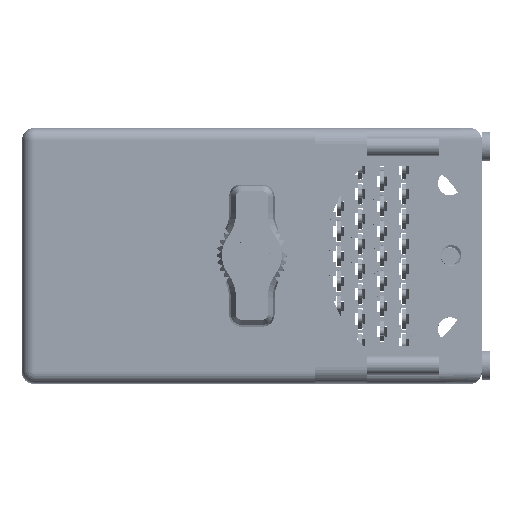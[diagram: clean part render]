
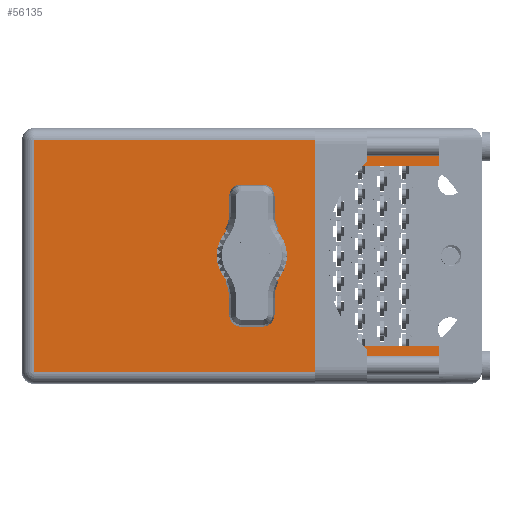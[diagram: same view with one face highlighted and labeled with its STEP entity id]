
A CAD part, top view. The second image highlights one B-rep face of the part: STEP entity #56135.
In plain terms, the highlighted face is planar.
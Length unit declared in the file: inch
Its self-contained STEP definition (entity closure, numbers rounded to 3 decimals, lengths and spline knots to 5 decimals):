
#214 = LINE ( 'NONE', #39672, #83314 ) ;
#845 = VERTEX_POINT ( 'NONE', #43709 ) ;
#1133 = EDGE_CURVE ( 'NONE', #43625, #47633, #113852, .T. ) ;
#6510 = DIRECTION ( 'NONE',  ( 0., 1., 0. ) ) ;
#6665 = EDGE_LOOP ( 'NONE', ( #37885, #8141 ) ) ;
#8141 = ORIENTED_EDGE ( 'NONE', *, *, #75667, .F. ) ;
#11729 = ORIENTED_EDGE ( 'NONE', *, *, #46398, .T. ) ;
#15214 = CIRCLE ( 'NONE', #17256, 0.17 ) ;
#16119 = CARTESIAN_POINT ( 'NONE',  ( 0., 2.03, -1.46 ) ) ;
#16270 = VECTOR ( 'NONE', #66486, 39.37008 ) ;
#17256 = AXIS2_PLACEMENT_3D ( 'NONE', #53500, #71880, #35400 ) ;
#17842 = CARTESIAN_POINT ( 'NONE',  ( 0.07, 2.03, -0.07 ) ) ;
#19711 = VERTEX_POINT ( 'NONE', #57983 ) ;
#20556 = EDGE_CURVE ( 'NONE', #73441, #50418, #86297, .T. ) ;
#21620 = CIRCLE ( 'NONE', #43722, 0.17 ) ;
#24631 = VECTOR ( 'NONE', #107066, 39.37008 ) ;
#25936 = ORIENTED_EDGE ( 'NONE', *, *, #43017, .T. ) ;
#27123 = VECTOR ( 'NONE', #75668, 39.37008 ) ;
#32045 = CARTESIAN_POINT ( 'NONE',  ( 2.499, 2.03, -1.46 ) ) ;
#35400 = DIRECTION ( 'NONE',  ( 0., 0., 1. ) ) ;
#35811 = ORIENTED_EDGE ( 'NONE', *, *, #83329, .T. ) ;
#37885 = ORIENTED_EDGE ( 'NONE', *, *, #70931, .F. ) ;
#38828 = CARTESIAN_POINT ( 'NONE',  ( 2.499, 2.03, -0.07 ) ) ;
#39672 = CARTESIAN_POINT ( 'NONE',  ( 1.785, 2.03, -1.305 ) ) ;
#40812 = FACE_BOUND ( 'NONE', #6665, .T. ) ;
#43017 = EDGE_CURVE ( 'NONE', #55716, #47633, #66844, .T. ) ;
#43625 = VERTEX_POINT ( 'NONE', #32045 ) ;
#43709 = CARTESIAN_POINT ( 'NONE',  ( 1.3775, 2.03, -0.935 ) ) ;
#43722 = AXIS2_PLACEMENT_3D ( 'NONE', #115340, #49992, #114144 ) ;
#46033 = VECTOR ( 'NONE', #117172, 39.37008 ) ;
#46398 = EDGE_CURVE ( 'NONE', #49380, #82780, #96384, .T. ) ;
#47633 = VERTEX_POINT ( 'NONE', #61844 ) ;
#49380 = VERTEX_POINT ( 'NONE', #49765 ) ;
#49470 = FACE_OUTER_BOUND ( 'NONE', #64217, .T. ) ;
#49765 = CARTESIAN_POINT ( 'NONE',  ( 0.07, 2.03, -1.46 ) ) ;
#49992 = DIRECTION ( 'NONE',  ( 0., 1., 0. ) ) ;
#50418 = VERTEX_POINT ( 'NONE', #77451 ) ;
#53500 = CARTESIAN_POINT ( 'NONE',  ( 1.3775, 2.03, -0.765 ) ) ;
#55258 = CARTESIAN_POINT ( 'NONE',  ( 2.499, 2.03, -0.225 ) ) ;
#55716 = VERTEX_POINT ( 'NONE', #75066 ) ;
#56135 = ADVANCED_FACE ( 'NONE', ( #49470, #40812 ), #116376, .T. ) ;
#57983 = CARTESIAN_POINT ( 'NONE',  ( 1.785, 2.03, -0.225 ) ) ;
#61399 = CARTESIAN_POINT ( 'NONE',  ( 0., 2.03, -1.53 ) ) ;
#61844 = CARTESIAN_POINT ( 'NONE',  ( 2.499, 2.03, -1.305 ) ) ;
#64217 = EDGE_LOOP ( 'NONE', ( #11729, #109467, #86239, #91679, #83997, #25936, #95914, #35811 ) ) ;
#66486 = DIRECTION ( 'NONE',  ( 0., 0., 1. ) ) ;
#66844 = LINE ( 'NONE', #75076, #104107 ) ;
#70622 = DIRECTION ( 'NONE',  ( 0., 0., 1. ) ) ;
#70931 = EDGE_CURVE ( 'NONE', #85404, #845, #15214, .T. ) ;
#71880 = DIRECTION ( 'NONE',  ( 0., 1., 0. ) ) ;
#73441 = VERTEX_POINT ( 'NONE', #55258 ) ;
#75066 = CARTESIAN_POINT ( 'NONE',  ( 1.785, 2.03, -1.305 ) ) ;
#75076 = CARTESIAN_POINT ( 'NONE',  ( 2.499, 2.03, -1.305 ) ) ;
#75667 = EDGE_CURVE ( 'NONE', #845, #85404, #21620, .T. ) ;
#75668 = DIRECTION ( 'NONE',  ( 1., 0., 0. ) ) ;
#77451 = CARTESIAN_POINT ( 'NONE',  ( 2.499, 2.03, -0.07 ) ) ;
#80508 = CARTESIAN_POINT ( 'NONE',  ( 0.07, 2.03, -1.53 ) ) ;
#81864 = LINE ( 'NONE', #16119, #46033 ) ;
#82780 = VERTEX_POINT ( 'NONE', #17842 ) ;
#83314 = VECTOR ( 'NONE', #113024, 39.37008 ) ;
#83329 = EDGE_CURVE ( 'NONE', #43625, #49380, #81864, .T. ) ;
#83997 = ORIENTED_EDGE ( 'NONE', *, *, #110821, .T. ) ;
#85404 = VERTEX_POINT ( 'NONE', #89742 ) ;
#86239 = ORIENTED_EDGE ( 'NONE', *, *, #20556, .F. ) ;
#86297 = LINE ( 'NONE', #106674, #24631 ) ;
#88904 = LINE ( 'NONE', #38828, #27123 ) ;
#89742 = CARTESIAN_POINT ( 'NONE',  ( 1.3775, 2.03, -0.595 ) ) ;
#91679 = ORIENTED_EDGE ( 'NONE', *, *, #94814, .T. ) ;
#92186 = LINE ( 'NONE', #95443, #97932 ) ;
#94814 = EDGE_CURVE ( 'NONE', #73441, #19711, #92186, .T. ) ;
#95443 = CARTESIAN_POINT ( 'NONE',  ( 2.499, 2.03, -0.225 ) ) ;
#95914 = ORIENTED_EDGE ( 'NONE', *, *, #1133, .F. ) ;
#96384 = LINE ( 'NONE', #80508, #104986 ) ;
#97932 = VECTOR ( 'NONE', #113921, 39.37008 ) ;
#98586 = DIRECTION ( 'NONE',  ( 0., 0., 1. ) ) ;
#99347 = AXIS2_PLACEMENT_3D ( 'NONE', #61399, #6510, #70622 ) ;
#104107 = VECTOR ( 'NONE', #115647, 39.37008 ) ;
#104145 = CARTESIAN_POINT ( 'NONE',  ( 2.499, 2.03, -1.53 ) ) ;
#104986 = VECTOR ( 'NONE', #98586, 39.37008 ) ;
#106674 = CARTESIAN_POINT ( 'NONE',  ( 2.499, 2.03, -1.53 ) ) ;
#107066 = DIRECTION ( 'NONE',  ( 0., 0., 1. ) ) ;
#109467 = ORIENTED_EDGE ( 'NONE', *, *, #118419, .T. ) ;
#110821 = EDGE_CURVE ( 'NONE', #19711, #55716, #214, .T. ) ;
#113024 = DIRECTION ( 'NONE',  ( 0., 0., -1. ) ) ;
#113852 = LINE ( 'NONE', #104145, #16270 ) ;
#113921 = DIRECTION ( 'NONE',  ( -1., 0., 0. ) ) ;
#114144 = DIRECTION ( 'NONE',  ( 0., 0., 1. ) ) ;
#115340 = CARTESIAN_POINT ( 'NONE',  ( 1.3775, 2.03, -0.765 ) ) ;
#115647 = DIRECTION ( 'NONE',  ( 1., 0., 0. ) ) ;
#116376 = PLANE ( 'NONE',  #99347 ) ;
#117172 = DIRECTION ( 'NONE',  ( -1., 0., 0. ) ) ;
#118419 = EDGE_CURVE ( 'NONE', #82780, #50418, #88904, .T. ) ;
